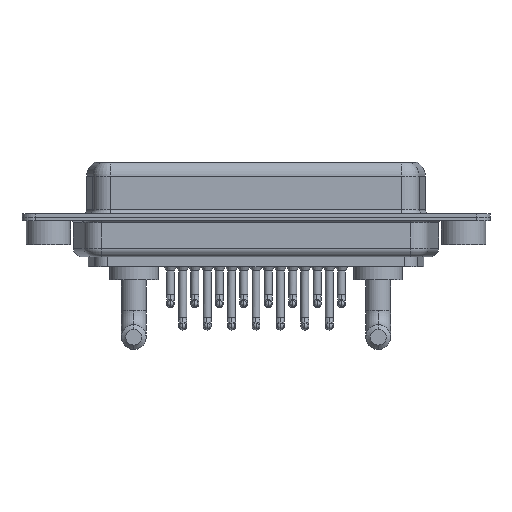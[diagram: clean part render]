
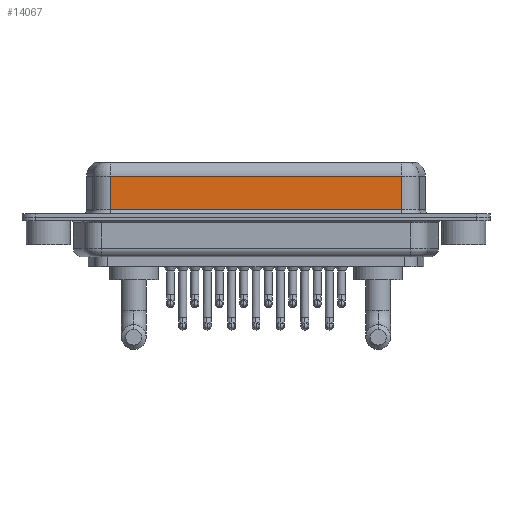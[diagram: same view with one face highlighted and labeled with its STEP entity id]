
A CAD part, front view. The second image highlights one B-rep face of the part: STEP entity #14067.
In plain terms, the highlighted planar face has unit normal (0, -1, 0).
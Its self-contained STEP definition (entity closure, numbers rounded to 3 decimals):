
#567 = EDGE_CURVE ( 'NONE', #7417, #1524, #2199, .T. ) ;
#1481 = CARTESIAN_POINT ( 'NONE',  ( 7.013, -3.95, 4.65 ) ) ;
#1524 = VERTEX_POINT ( 'NONE', #1481 ) ;
#2199 = LINE ( 'NONE', #8679, #8000 ) ;
#2667 = VERTEX_POINT ( 'NONE', #4933 ) ;
#2998 = DIRECTION ( 'NONE',  ( 0., 0., -1. ) ) ;
#3149 = EDGE_CURVE ( 'NONE', #7417, #17035, #6300, .T. ) ;
#3536 = VECTOR ( 'NONE', #2998, 1000. ) ;
#3662 = CARTESIAN_POINT ( 'NONE',  ( 7.013, -3.95, 6.4 ) ) ;
#3870 = LINE ( 'NONE', #3662, #12394 ) ;
#4933 = CARTESIAN_POINT ( 'NONE',  ( 7.013, -3.95, 0.9 ) ) ;
#5286 = EDGE_CURVE ( 'NONE', #2667, #17035, #7734, .T. ) ;
#6300 = LINE ( 'NONE', #14446, #3536 ) ;
#7017 = CARTESIAN_POINT ( 'NONE',  ( 40.037, -3.95, 4.65 ) ) ;
#7261 = DIRECTION ( 'NONE',  ( 0., 0., 1. ) ) ;
#7417 = VERTEX_POINT ( 'NONE', #7017 ) ;
#7734 = LINE ( 'NONE', #10789, #11922 ) ;
#8000 = VECTOR ( 'NONE', #20069, 1000. ) ;
#8679 = CARTESIAN_POINT ( 'NONE',  ( 40.037, -3.95, 4.65 ) ) ;
#9875 = ORIENTED_EDGE ( 'NONE', *, *, #12113, .T. ) ;
#10789 = CARTESIAN_POINT ( 'NONE',  ( 40.037, -3.95, 0.9 ) ) ;
#11922 = VECTOR ( 'NONE', #12593, 1000. ) ;
#12113 = EDGE_CURVE ( 'NONE', #1524, #2667, #3870, .T. ) ;
#12394 = VECTOR ( 'NONE', #16454, 1000. ) ;
#12593 = DIRECTION ( 'NONE',  ( 1., 0., 0. ) ) ;
#13707 = PLANE ( 'NONE',  #15841 ) ;
#14067 = ADVANCED_FACE ( 'NONE', ( #17174 ), #13707, .F. ) ;
#14446 = CARTESIAN_POINT ( 'NONE',  ( 40.037, -3.95, 6.4 ) ) ;
#15559 = CARTESIAN_POINT ( 'NONE',  ( 40.037, -3.95, 0.9 ) ) ;
#15841 = AXIS2_PLACEMENT_3D ( 'NONE', #17065, #18453, #7261 ) ;
#16454 = DIRECTION ( 'NONE',  ( 0., 0., -1. ) ) ;
#16541 = ORIENTED_EDGE ( 'NONE', *, *, #3149, .F. ) ;
#16645 = EDGE_LOOP ( 'NONE', ( #16541, #16877, #9875, #19726 ) ) ;
#16877 = ORIENTED_EDGE ( 'NONE', *, *, #567, .T. ) ;
#17035 = VERTEX_POINT ( 'NONE', #15559 ) ;
#17065 = CARTESIAN_POINT ( 'NONE',  ( 40.037, -3.95, 6.4 ) ) ;
#17174 = FACE_OUTER_BOUND ( 'NONE', #16645, .T. ) ;
#18453 = DIRECTION ( 'NONE',  ( 0., 1., 0. ) ) ;
#19726 = ORIENTED_EDGE ( 'NONE', *, *, #5286, .T. ) ;
#20069 = DIRECTION ( 'NONE',  ( -1., 0., 0. ) ) ;
